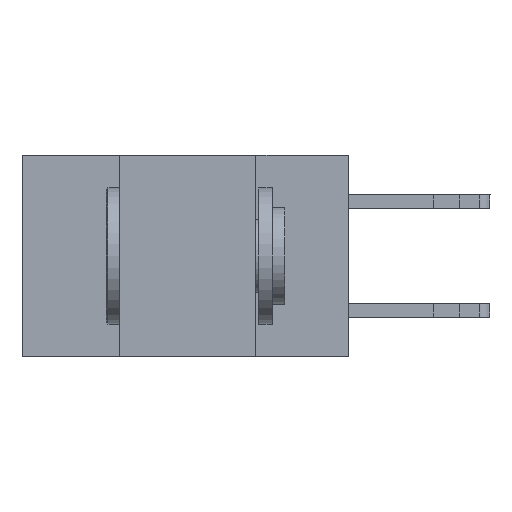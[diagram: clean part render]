
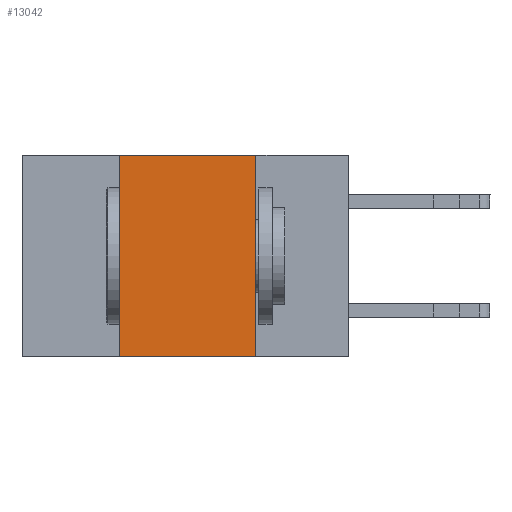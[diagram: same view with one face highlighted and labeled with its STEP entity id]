
A CAD part, left-side view. The second image highlights one B-rep face of the part: STEP entity #13042.
In plain terms, the highlighted planar face has unit normal (-1, 0, 0).
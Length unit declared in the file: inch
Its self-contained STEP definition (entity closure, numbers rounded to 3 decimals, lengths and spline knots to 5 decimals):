
#11 = DIRECTION ( 'NONE',  ( 0., 0., 1. ) ) ;
#613 = EDGE_LOOP ( 'NONE', ( #9312, #15645, #1670, #14361 ) ) ;
#614 = LINE ( 'NONE', #4755, #10535 ) ;
#623 = LINE ( 'NONE', #800, #7948 ) ;
#800 = CARTESIAN_POINT ( 'NONE',  ( 0., 0.6, 0. ) ) ;
#880 = CARTESIAN_POINT ( 'NONE',  ( 0., 0.17, 0. ) ) ;
#1670 = ORIENTED_EDGE ( 'NONE', *, *, #6450, .F. ) ;
#2996 = EDGE_CURVE ( 'NONE', #10616, #13238, #623, .T. ) ;
#3058 = FACE_OUTER_BOUND ( 'NONE', #613, .T. ) ;
#3240 = CARTESIAN_POINT ( 'NONE',  ( 0., 0.6, 0. ) ) ;
#3323 = PLANE ( 'NONE',  #7430 ) ;
#3341 = VECTOR ( 'NONE', #11, 39.37008 ) ;
#4422 = CARTESIAN_POINT ( 'NONE',  ( 0., 0.42, 0. ) ) ;
#4653 = LINE ( 'NONE', #11488, #14922 ) ;
#4755 = CARTESIAN_POINT ( 'NONE',  ( 0., 0.17, 0. ) ) ;
#5942 = DIRECTION ( 'NONE',  ( 0., 0., -1. ) ) ;
#6450 = EDGE_CURVE ( 'NONE', #13513, #10616, #9745, .T. ) ;
#7112 = DIRECTION ( 'NONE',  ( 1., 0., 0. ) ) ;
#7430 = AXIS2_PLACEMENT_3D ( 'NONE', #3240, #7112, #5942 ) ;
#7948 = VECTOR ( 'NONE', #11596, 39.37008 ) ;
#8617 = CARTESIAN_POINT ( 'NONE',  ( 0., 0.42, -0.37 ) ) ;
#9312 = ORIENTED_EDGE ( 'NONE', *, *, #10543, .F. ) ;
#9745 = LINE ( 'NONE', #4422, #3341 ) ;
#10535 = VECTOR ( 'NONE', #14578, 39.37008 ) ;
#10543 = EDGE_CURVE ( 'NONE', #13238, #14171, #614, .T. ) ;
#10616 = VERTEX_POINT ( 'NONE', #11191 ) ;
#11191 = CARTESIAN_POINT ( 'NONE',  ( 0., 0.42, 0. ) ) ;
#11488 = CARTESIAN_POINT ( 'NONE',  ( 0., 0.6, -0.37 ) ) ;
#11596 = DIRECTION ( 'NONE',  ( 0., -1., 0. ) ) ;
#12262 = CARTESIAN_POINT ( 'NONE',  ( 0., 0.17, -0.37 ) ) ;
#13042 = ADVANCED_FACE ( 'NONE', ( #3058 ), #3323, .F. ) ;
#13238 = VERTEX_POINT ( 'NONE', #880 ) ;
#13426 = EDGE_CURVE ( 'NONE', #13513, #14171, #4653, .T. ) ;
#13513 = VERTEX_POINT ( 'NONE', #8617 ) ;
#14171 = VERTEX_POINT ( 'NONE', #12262 ) ;
#14361 = ORIENTED_EDGE ( 'NONE', *, *, #13426, .T. ) ;
#14578 = DIRECTION ( 'NONE',  ( 0., 0., -1. ) ) ;
#14922 = VECTOR ( 'NONE', #16823, 39.37008 ) ;
#15645 = ORIENTED_EDGE ( 'NONE', *, *, #2996, .F. ) ;
#16823 = DIRECTION ( 'NONE',  ( 0., -1., 0. ) ) ;
